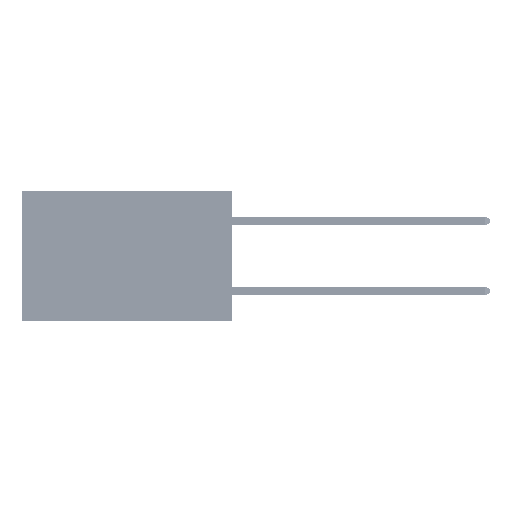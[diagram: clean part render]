
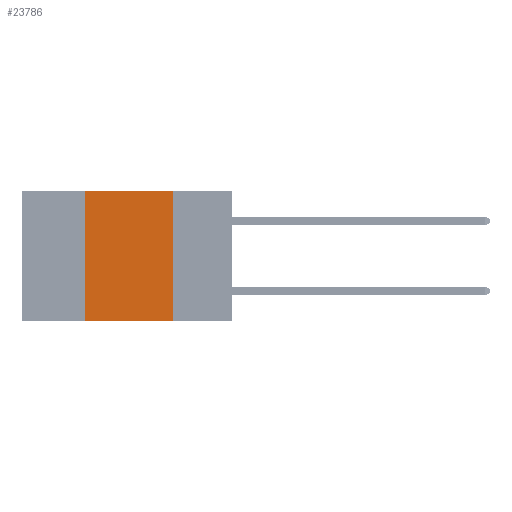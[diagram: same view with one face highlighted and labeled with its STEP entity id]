
A CAD part, left-side view. The second image highlights one B-rep face of the part: STEP entity #23786.
In plain terms, the highlighted planar face has unit normal (-1, 0, 0).
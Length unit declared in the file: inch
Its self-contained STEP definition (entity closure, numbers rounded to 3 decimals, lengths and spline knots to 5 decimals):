
#402 = CARTESIAN_POINT ( 'NONE',  ( 0., 0.42, 0. ) ) ;
#2213 = VERTEX_POINT ( 'NONE', #17070 ) ;
#4826 = VERTEX_POINT ( 'NONE', #36538 ) ;
#11357 = VECTOR ( 'NONE', #28109, 39.37008 ) ;
#12267 = EDGE_LOOP ( 'NONE', ( #14183, #36850, #37187, #17430 ) ) ;
#12517 = EDGE_CURVE ( 'NONE', #20965, #4826, #48475, .T. ) ;
#14183 = ORIENTED_EDGE ( 'NONE', *, *, #41468, .F. ) ;
#15209 = DIRECTION ( 'NONE',  ( 0., 0., 1. ) ) ;
#17070 = CARTESIAN_POINT ( 'NONE',  ( 0., 0.17, -0.37 ) ) ;
#17430 = ORIENTED_EDGE ( 'NONE', *, *, #36323, .T. ) ;
#18325 = DIRECTION ( 'NONE',  ( 0., 0., -1. ) ) ;
#19084 = DIRECTION ( 'NONE',  ( 0., -1., 0. ) ) ;
#19975 = LINE ( 'NONE', #48596, #32328 ) ;
#19979 = AXIS2_PLACEMENT_3D ( 'NONE', #37524, #26024, #18325 ) ;
#20965 = VERTEX_POINT ( 'NONE', #44224 ) ;
#21003 = VECTOR ( 'NONE', #27626, 39.37008 ) ;
#23786 = ADVANCED_FACE ( 'NONE', ( #41081 ), #36875, .F. ) ;
#24513 = CARTESIAN_POINT ( 'NONE',  ( 0., 0.6, -0.37 ) ) ;
#26024 = DIRECTION ( 'NONE',  ( 1., 0., 0. ) ) ;
#26876 = LINE ( 'NONE', #42578, #21003 ) ;
#27452 = CARTESIAN_POINT ( 'NONE',  ( 0., 0.17, 0. ) ) ;
#27626 = DIRECTION ( 'NONE',  ( 0., 0., -1. ) ) ;
#28109 = DIRECTION ( 'NONE',  ( 0., -1., 0. ) ) ;
#30948 = EDGE_CURVE ( 'NONE', #4826, #48270, #19975, .T. ) ;
#32328 = VECTOR ( 'NONE', #19084, 39.37008 ) ;
#33111 = LINE ( 'NONE', #24513, #11357 ) ;
#36323 = EDGE_CURVE ( 'NONE', #20965, #2213, #33111, .T. ) ;
#36538 = CARTESIAN_POINT ( 'NONE',  ( 0., 0.42, 0. ) ) ;
#36850 = ORIENTED_EDGE ( 'NONE', *, *, #30948, .F. ) ;
#36875 = PLANE ( 'NONE',  #19979 ) ;
#37187 = ORIENTED_EDGE ( 'NONE', *, *, #12517, .F. ) ;
#37524 = CARTESIAN_POINT ( 'NONE',  ( 0., 0.6, 0. ) ) ;
#41081 = FACE_OUTER_BOUND ( 'NONE', #12267, .T. ) ;
#41468 = EDGE_CURVE ( 'NONE', #48270, #2213, #26876, .T. ) ;
#42578 = CARTESIAN_POINT ( 'NONE',  ( 0., 0.17, 0. ) ) ;
#44224 = CARTESIAN_POINT ( 'NONE',  ( 0., 0.42, -0.37 ) ) ;
#47867 = VECTOR ( 'NONE', #15209, 39.37008 ) ;
#48270 = VERTEX_POINT ( 'NONE', #27452 ) ;
#48475 = LINE ( 'NONE', #402, #47867 ) ;
#48596 = CARTESIAN_POINT ( 'NONE',  ( 0., 0.6, 0. ) ) ;
